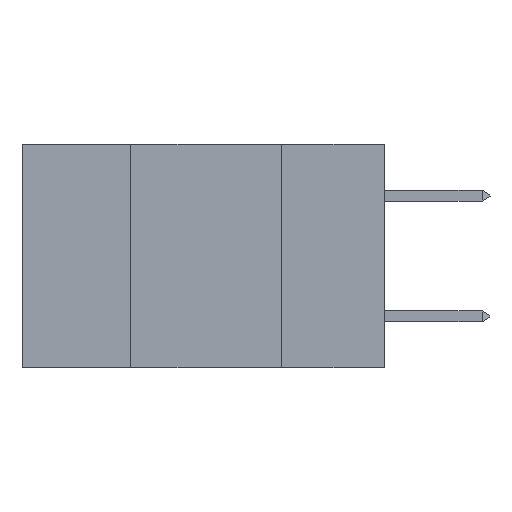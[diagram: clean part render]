
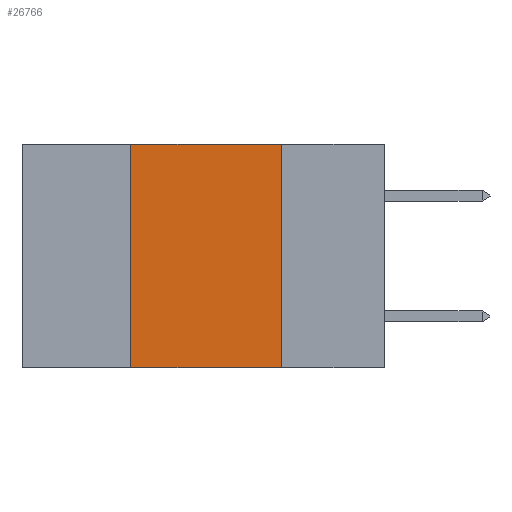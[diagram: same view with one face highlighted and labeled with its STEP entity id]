
A CAD part, left-side view. The second image highlights one B-rep face of the part: STEP entity #26766.
In plain terms, the highlighted planar face has unit normal (-1, 0, 0).
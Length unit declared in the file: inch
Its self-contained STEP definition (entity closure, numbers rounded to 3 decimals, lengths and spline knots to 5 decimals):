
#678 = CARTESIAN_POINT ( 'NONE',  ( 0., 0.42, -0.37 ) ) ;
#1890 = PLANE ( 'NONE',  #14912 ) ;
#2184 = FACE_OUTER_BOUND ( 'NONE', #13256, .T. ) ;
#3129 = ORIENTED_EDGE ( 'NONE', *, *, #12485, .F. ) ;
#3727 = VECTOR ( 'NONE', #28850, 39.37008 ) ;
#4441 = DIRECTION ( 'NONE',  ( 0., 0., -1. ) ) ;
#4514 = EDGE_CURVE ( 'NONE', #15491, #20762, #12268, .T. ) ;
#5407 = ORIENTED_EDGE ( 'NONE', *, *, #4514, .F. ) ;
#8969 = CARTESIAN_POINT ( 'NONE',  ( 0., 0.6, 0. ) ) ;
#9296 = VECTOR ( 'NONE', #27234, 39.37008 ) ;
#10458 = CARTESIAN_POINT ( 'NONE',  ( 0., 0.6, 0. ) ) ;
#11201 = VECTOR ( 'NONE', #28027, 39.37008 ) ;
#11763 = LINE ( 'NONE', #18975, #16658 ) ;
#12268 = LINE ( 'NONE', #10458, #3727 ) ;
#12345 = LINE ( 'NONE', #18824, #11201 ) ;
#12485 = EDGE_CURVE ( 'NONE', #25602, #15491, #12345, .T. ) ;
#12861 = EDGE_CURVE ( 'NONE', #25602, #14370, #23030, .T. ) ;
#13256 = EDGE_LOOP ( 'NONE', ( #20091, #5407, #3129, #17668 ) ) ;
#13390 = CARTESIAN_POINT ( 'NONE',  ( 0., 0.6, -0.37 ) ) ;
#14370 = VERTEX_POINT ( 'NONE', #16114 ) ;
#14912 = AXIS2_PLACEMENT_3D ( 'NONE', #8969, #15885, #4441 ) ;
#15491 = VERTEX_POINT ( 'NONE', #15678 ) ;
#15678 = CARTESIAN_POINT ( 'NONE',  ( 0., 0.42, 0. ) ) ;
#15885 = DIRECTION ( 'NONE',  ( 1., 0., 0. ) ) ;
#16114 = CARTESIAN_POINT ( 'NONE',  ( 0., 0.17, -0.37 ) ) ;
#16658 = VECTOR ( 'NONE', #25916, 39.37008 ) ;
#17022 = EDGE_CURVE ( 'NONE', #20762, #14370, #11763, .T. ) ;
#17668 = ORIENTED_EDGE ( 'NONE', *, *, #12861, .T. ) ;
#18824 = CARTESIAN_POINT ( 'NONE',  ( 0., 0.42, 0. ) ) ;
#18975 = CARTESIAN_POINT ( 'NONE',  ( 0., 0.17, 0. ) ) ;
#19637 = CARTESIAN_POINT ( 'NONE',  ( 0., 0.17, 0. ) ) ;
#20091 = ORIENTED_EDGE ( 'NONE', *, *, #17022, .F. ) ;
#20762 = VERTEX_POINT ( 'NONE', #19637 ) ;
#23030 = LINE ( 'NONE', #13390, #9296 ) ;
#25602 = VERTEX_POINT ( 'NONE', #678 ) ;
#25916 = DIRECTION ( 'NONE',  ( 0., 0., -1. ) ) ;
#26766 = ADVANCED_FACE ( 'NONE', ( #2184 ), #1890, .F. ) ;
#27234 = DIRECTION ( 'NONE',  ( 0., -1., 0. ) ) ;
#28027 = DIRECTION ( 'NONE',  ( 0., 0., 1. ) ) ;
#28850 = DIRECTION ( 'NONE',  ( 0., -1., 0. ) ) ;
